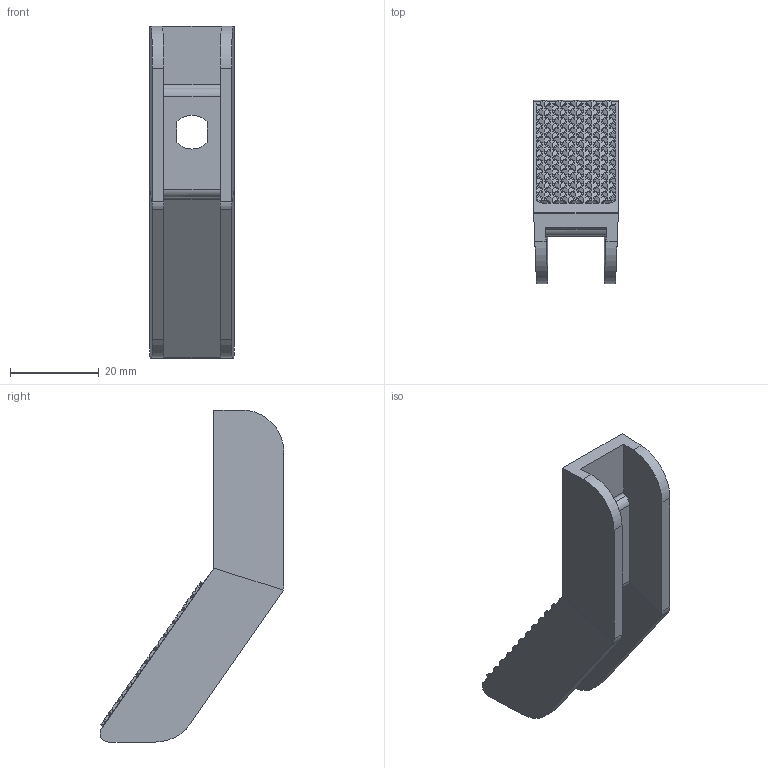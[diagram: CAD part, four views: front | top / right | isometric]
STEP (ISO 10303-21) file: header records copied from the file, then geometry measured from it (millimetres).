
FILE_DESCRIPTION (( 'STEP AP214' ), '1' );
FILE_NAME ('User Library-Telescopic Stock_Telescopic Stock Lever1.STEP', '2013-05-23T12:57:33', ( 'Asher' ), ( '' ), 'SwSTEP 2.0', 'SolidWorks 2013', '' );
FILE_SCHEMA (( 'AUTOMOTIVE_DESIGN' ));
Length unit declared in the file: millimetre
Products named in the file (1): User Library-Telescopic Stock_Telescopic Stock Lever1
Bounding box: 19.05 x 41.36 x 74.68 mm (x, y, z)
Volume: 10694.9 mm3; surface area: 8125.3 mm2
Topology: 1 solids, 1 shells, 643 faces, 1545 edges, 1030 vertices
Faces by surface type: plane 620, cylinder 23
Entity records: 18339 total; most frequent: CARTESIAN_POINT 3339, ORIENTED_EDGE 3090, DIRECTION 2815, EDGE_CURVE 1545, LINE 1483, VECTOR 1483, VERTEX_POINT 1030, EDGE_LOOP 771
